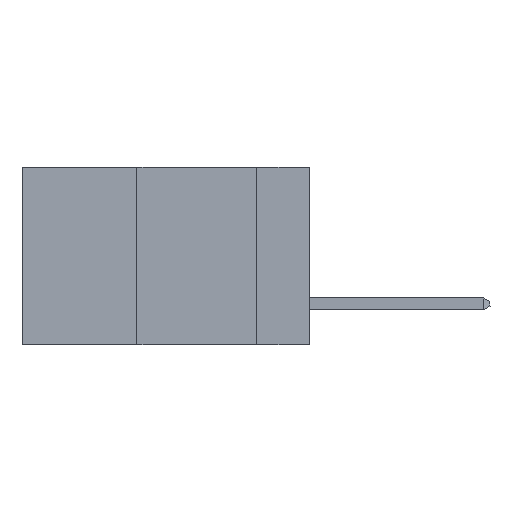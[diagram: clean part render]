
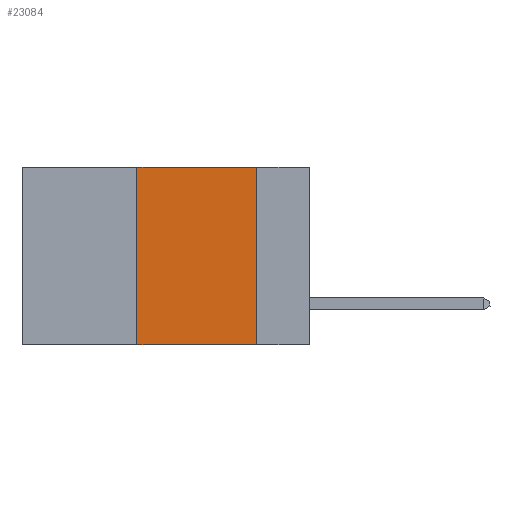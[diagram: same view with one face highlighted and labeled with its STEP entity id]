
A CAD part, left-side view. The second image highlights one B-rep face of the part: STEP entity #23084.
In plain terms, the highlighted planar face has unit normal (-1, 0, 0).
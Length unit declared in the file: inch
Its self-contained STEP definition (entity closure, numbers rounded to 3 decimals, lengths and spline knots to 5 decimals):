
#208 = EDGE_CURVE ( 'NONE', #5750, #4458, #9318, .T. ) ;
#599 = AXIS2_PLACEMENT_3D ( 'NONE', #24024, #4827, #18421 ) ;
#954 = DIRECTION ( 'NONE',  ( 0., 0., -1. ) ) ;
#968 = PLANE ( 'NONE',  #599 ) ;
#1401 = VECTOR ( 'NONE', #954, 39.37008 ) ;
#1457 = VECTOR ( 'NONE', #13430, 39.37008 ) ;
#2705 = ORIENTED_EDGE ( 'NONE', *, *, #12754, .T. ) ;
#4458 = VERTEX_POINT ( 'NONE', #14053 ) ;
#4555 = CARTESIAN_POINT ( 'NONE',  ( 0., 0.36, 0. ) ) ;
#4778 = CARTESIAN_POINT ( 'NONE',  ( 0., 0.11, -0.37 ) ) ;
#4827 = DIRECTION ( 'NONE',  ( 1., 0., 0. ) ) ;
#5461 = CARTESIAN_POINT ( 'NONE',  ( 0., 0.11, 0. ) ) ;
#5750 = VERTEX_POINT ( 'NONE', #13245 ) ;
#8694 = VECTOR ( 'NONE', #15058, 39.37008 ) ;
#9318 = LINE ( 'NONE', #4555, #8694 ) ;
#10473 = LINE ( 'NONE', #21513, #20127 ) ;
#11357 = CARTESIAN_POINT ( 'NONE',  ( 0., 0.6, 0. ) ) ;
#12305 = EDGE_CURVE ( 'NONE', #23944, #13027, #21326, .T. ) ;
#12754 = EDGE_CURVE ( 'NONE', #5750, #13027, #10473, .T. ) ;
#13027 = VERTEX_POINT ( 'NONE', #4778 ) ;
#13245 = CARTESIAN_POINT ( 'NONE',  ( 0., 0.36, -0.37 ) ) ;
#13430 = DIRECTION ( 'NONE',  ( 0., -1., 0. ) ) ;
#14053 = CARTESIAN_POINT ( 'NONE',  ( 0., 0.36, 0. ) ) ;
#15058 = DIRECTION ( 'NONE',  ( 0., 0., 1. ) ) ;
#15738 = EDGE_LOOP ( 'NONE', ( #23246, #19133, #21441, #2705 ) ) ;
#16949 = LINE ( 'NONE', #11357, #1457 ) ;
#17992 = FACE_OUTER_BOUND ( 'NONE', #15738, .T. ) ;
#18421 = DIRECTION ( 'NONE',  ( 0., 0., -1. ) ) ;
#18703 = EDGE_CURVE ( 'NONE', #4458, #23944, #16949, .T. ) ;
#19133 = ORIENTED_EDGE ( 'NONE', *, *, #18703, .F. ) ;
#20127 = VECTOR ( 'NONE', #23413, 39.37008 ) ;
#20227 = CARTESIAN_POINT ( 'NONE',  ( 0., 0.11, 0. ) ) ;
#21326 = LINE ( 'NONE', #20227, #1401 ) ;
#21441 = ORIENTED_EDGE ( 'NONE', *, *, #208, .F. ) ;
#21513 = CARTESIAN_POINT ( 'NONE',  ( 0., 0.6, -0.37 ) ) ;
#23084 = ADVANCED_FACE ( 'NONE', ( #17992 ), #968, .F. ) ;
#23246 = ORIENTED_EDGE ( 'NONE', *, *, #12305, .F. ) ;
#23413 = DIRECTION ( 'NONE',  ( 0., -1., 0. ) ) ;
#23944 = VERTEX_POINT ( 'NONE', #5461 ) ;
#24024 = CARTESIAN_POINT ( 'NONE',  ( 0., 0.6, 0. ) ) ;
